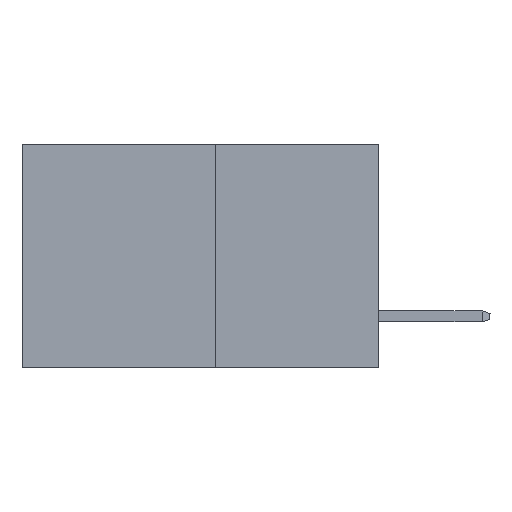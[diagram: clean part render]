
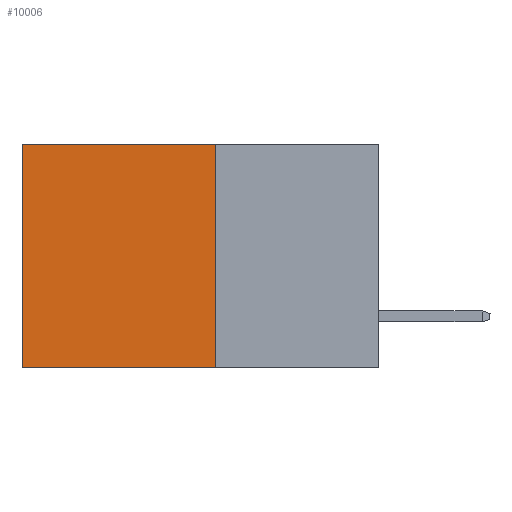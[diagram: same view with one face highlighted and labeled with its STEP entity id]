
A CAD part, left-side view. The second image highlights one B-rep face of the part: STEP entity #10006.
In plain terms, the highlighted planar face has unit normal (-1, 0, 0).
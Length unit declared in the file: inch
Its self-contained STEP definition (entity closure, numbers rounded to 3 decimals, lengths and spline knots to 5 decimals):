
#144 = VERTEX_POINT ( 'NONE', #4758 ) ;
#543 = DIRECTION ( 'NONE',  ( 0., 0., -1. ) ) ;
#767 = EDGE_CURVE ( 'NONE', #4547, #144, #13305, .T. ) ;
#1533 = CARTESIAN_POINT ( 'NONE',  ( 0.277, 0.59, -0.37 ) ) ;
#2258 = EDGE_LOOP ( 'NONE', ( #14630, #6128, #11177, #12253 ) ) ;
#3633 = VERTEX_POINT ( 'NONE', #20172 ) ;
#4547 = VERTEX_POINT ( 'NONE', #16839 ) ;
#4758 = CARTESIAN_POINT ( 'NONE',  ( 0.277, 0.27, -0.37 ) ) ;
#5117 = DIRECTION ( 'NONE',  ( 0., 0., -1. ) ) ;
#5122 = DIRECTION ( 'NONE',  ( 1., 0., 0. ) ) ;
#5168 = CARTESIAN_POINT ( 'NONE',  ( 0.277, 0.27, -0.37 ) ) ;
#5194 = PLANE ( 'NONE',  #19527 ) ;
#5358 = VECTOR ( 'NONE', #543, 39.37008 ) ;
#6128 = ORIENTED_EDGE ( 'NONE', *, *, #9298, .F. ) ;
#7460 = LINE ( 'NONE', #14290, #16519 ) ;
#7837 = EDGE_CURVE ( 'NONE', #8026, #3633, #13842, .T. ) ;
#8026 = VERTEX_POINT ( 'NONE', #16205 ) ;
#9298 = EDGE_CURVE ( 'NONE', #144, #3633, #10069, .T. ) ;
#10006 = ADVANCED_FACE ( 'NONE', ( #17244 ), #5194, .F. ) ;
#10069 = LINE ( 'NONE', #12800, #13520 ) ;
#11177 = ORIENTED_EDGE ( 'NONE', *, *, #767, .F. ) ;
#12253 = ORIENTED_EDGE ( 'NONE', *, *, #19352, .T. ) ;
#12779 = DIRECTION ( 'NONE',  ( 0., 1., 0. ) ) ;
#12800 = CARTESIAN_POINT ( 'NONE',  ( 0.277, 0.27, -0.37 ) ) ;
#13305 = LINE ( 'NONE', #21851, #21687 ) ;
#13520 = VECTOR ( 'NONE', #12779, 39.37008 ) ;
#13842 = LINE ( 'NONE', #1533, #5358 ) ;
#14290 = CARTESIAN_POINT ( 'NONE',  ( 0.277, 0.27, 0. ) ) ;
#14630 = ORIENTED_EDGE ( 'NONE', *, *, #7837, .T. ) ;
#16018 = DIRECTION ( 'NONE',  ( 0., 1., 0. ) ) ;
#16205 = CARTESIAN_POINT ( 'NONE',  ( 0.277, 0.59, 0. ) ) ;
#16519 = VECTOR ( 'NONE', #16018, 39.37008 ) ;
#16839 = CARTESIAN_POINT ( 'NONE',  ( 0.277, 0.27, 0. ) ) ;
#17244 = FACE_OUTER_BOUND ( 'NONE', #2258, .T. ) ;
#17549 = DIRECTION ( 'NONE',  ( 0., 0., -1. ) ) ;
#19352 = EDGE_CURVE ( 'NONE', #4547, #8026, #7460, .T. ) ;
#19527 = AXIS2_PLACEMENT_3D ( 'NONE', #5168, #5122, #5117 ) ;
#20172 = CARTESIAN_POINT ( 'NONE',  ( 0.277, 0.59, -0.37 ) ) ;
#21687 = VECTOR ( 'NONE', #17549, 39.37008 ) ;
#21851 = CARTESIAN_POINT ( 'NONE',  ( 0.277, 0.27, -0.37 ) ) ;
